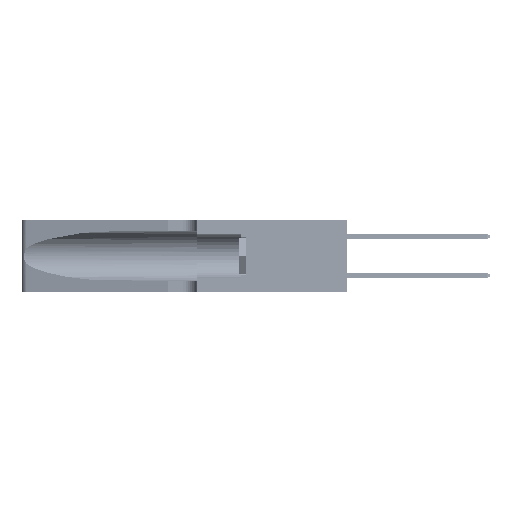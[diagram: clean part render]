
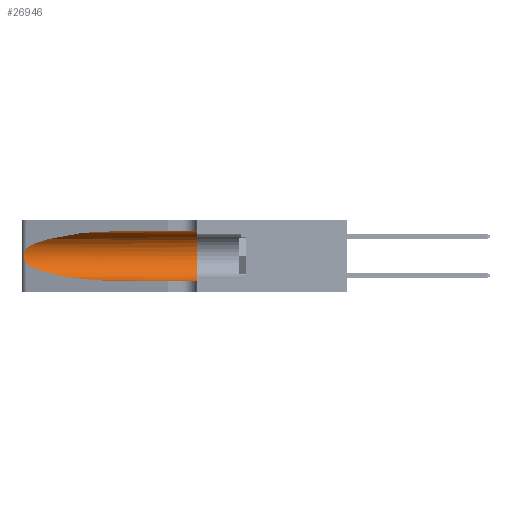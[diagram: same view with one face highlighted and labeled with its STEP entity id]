
A CAD part, left-side view. The second image highlights one B-rep face of the part: STEP entity #26946.
In plain terms, the highlighted cylindrical face has radius 3.308 mm (diameter 6.617 mm), a partial arc.
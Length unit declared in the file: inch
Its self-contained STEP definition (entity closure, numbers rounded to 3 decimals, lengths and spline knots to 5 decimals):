
#239 = VERTEX_POINT ( 'NONE', #35683 ) ;
#592 = CARTESIAN_POINT ( 'NONE',  ( 0.1305, 0.72297, 0.31525 ) ) ;
#1449 = ORIENTED_EDGE ( 'NONE', *, *, #2197, .T. ) ;
#1639 = DIRECTION ( 'NONE',  ( 0., 0., -1. ) ) ;
#1940 = VERTEX_POINT ( 'NONE', #25995 ) ;
#2197 = EDGE_CURVE ( 'NONE', #39018, #12454, #44494, .T. ) ;
#3047 = CARTESIAN_POINT ( 'NONE',  ( 0.25639, 1.23184, 0.21858 ) ) ;
#3977 = CARTESIAN_POINT ( 'NONE',  ( 0.25487, 1.22718, 0.14631 ) ) ;
#7223 = CARTESIAN_POINT ( 'NONE',  ( 0.25854, 1.2359, 0.20912 ) ) ;
#11367 = CARTESIAN_POINT ( 'NONE',  ( 0.26075, 1.23896, 0.19203 ) ) ;
#11879 =( BOUNDED_CURVE ( )  B_SPLINE_CURVE ( 3, ( #39941, #52371, #48402, #23644 ),
 .UNSPECIFIED., .F., .F. ) 
 B_SPLINE_CURVE_WITH_KNOTS ( ( 4, 4 ),
 ( 3.44316, 4.71239 ),
 .UNSPECIFIED. ) 
 CURVE ( )  GEOMETRIC_REPRESENTATION_ITEM ( )  RATIONAL_B_SPLINE_CURVE ( ( 1., 0.87, 0.87, 1. ) ) 
 REPRESENTATION_ITEM ( '' )  );
#12454 = VERTEX_POINT ( 'NONE', #33101 ) ;
#12565 = ORIENTED_EDGE ( 'NONE', *, *, #51630, .F. ) ;
#13204 = AXIS2_PLACEMENT_3D ( 'NONE', #22966, #51884, #27144 ) ;
#14034 = CYLINDRICAL_SURFACE ( 'NONE', #30666, 0.13025 ) ;
#15521 = CARTESIAN_POINT ( 'NONE',  ( 0.26017, 1.23833, 0.17102 ) ) ;
#16497 = CARTESIAN_POINT ( 'NONE',  ( 0.1305, 1.61858, 0.05475 ) ) ;
#18118 = CARTESIAN_POINT ( 'NONE',  ( 0.1305, 1.61858, 0.185 ) ) ;
#19456 = CARTESIAN_POINT ( 'NONE',  ( 0.1305, 0.72297, 0.31525 ) ) ;
#19464 = CARTESIAN_POINT ( 'NONE',  ( 0.25555, 1.22994, 0.2215 ) ) ;
#19646 = CARTESIAN_POINT ( 'NONE',  ( 0.25789, 1.23486, 0.15765 ) ) ;
#19848 = DIRECTION ( 'NONE',  ( 0., -1., 0. ) ) ;
#21571 = ORIENTED_EDGE ( 'NONE', *, *, #47830, .F. ) ;
#22966 = CARTESIAN_POINT ( 'NONE',  ( 0.1305, 0.35, 0.185 ) ) ;
#23084 = B_SPLINE_CURVE_WITH_KNOTS ( 'NONE', 3,
 ( #48365, #19464, #3047, #31985, #7223, #36110, #11367, #40264, #15521, #44382, #19646, #48542, #23790, #52678 ),
 .UNSPECIFIED., .F., .F.,
 ( 4, 2, 2, 2, 2, 2, 4 ),
 ( 0., 0.00027, 0.00053, 0.00107, 0.0016, 0.00187, 0.00214 ),
 .UNSPECIFIED. ) ;
#23644 = CARTESIAN_POINT ( 'NONE',  ( 0.1305, 0.72297, 0.05475 ) ) ;
#23790 = CARTESIAN_POINT ( 'NONE',  ( 0.25555, 1.22993, 0.14849 ) ) ;
#25995 = CARTESIAN_POINT ( 'NONE',  ( 0.1305, 0.35, 0.31525 ) ) ;
#26430 = DIRECTION ( 'NONE',  ( 0., -1., 0. ) ) ;
#26946 = ADVANCED_FACE ( 'NONE', ( #37276 ), #14034, .F. ) ;
#27144 = DIRECTION ( 'NONE',  ( 0., 0., 1. ) ) ;
#29186 = EDGE_CURVE ( 'NONE', #12454, #50051, #23084, .T. ) ;
#30012 = VECTOR ( 'NONE', #53472, 39.37008 ) ;
#30666 = AXIS2_PLACEMENT_3D ( 'NONE', #18118, #26430, #1639 ) ;
#31324 = LINE ( 'NONE', #16497, #30012 ) ;
#31796 = CARTESIAN_POINT ( 'NONE',  ( 0.2373, 1.15595, 0.28018 ) ) ;
#31985 = CARTESIAN_POINT ( 'NONE',  ( 0.25787, 1.23484, 0.2124 ) ) ;
#32183 = CARTESIAN_POINT ( 'NONE',  ( 0.1305, 1.61858, 0.31525 ) ) ;
#33101 = CARTESIAN_POINT ( 'NONE',  ( 0.25487, 1.22718, 0.22369 ) ) ;
#33103 = VECTOR ( 'NONE', #19848, 39.37008 ) ;
#33490 = EDGE_LOOP ( 'NONE', ( #1449, #34465, #49319, #40314, #12565, #21571 ) ) ;
#34465 = ORIENTED_EDGE ( 'NONE', *, *, #29186, .T. ) ;
#35683 = CARTESIAN_POINT ( 'NONE',  ( 0.1305, 0.72297, 0.05475 ) ) ;
#36110 = CARTESIAN_POINT ( 'NONE',  ( 0.26018, 1.23835, 0.19895 ) ) ;
#37189 = EDGE_CURVE ( 'NONE', #50051, #239, #11879, .T. ) ;
#37276 = FACE_OUTER_BOUND ( 'NONE', #33490, .T. ) ;
#39018 = VERTEX_POINT ( 'NONE', #592 ) ;
#39941 = CARTESIAN_POINT ( 'NONE',  ( 0.25487, 1.22718, 0.14631 ) ) ;
#40072 = CARTESIAN_POINT ( 'NONE',  ( 0.18966, 0.96281, 0.31525 ) ) ;
#40264 = CARTESIAN_POINT ( 'NONE',  ( 0.26075, 1.23896, 0.178 ) ) ;
#40314 = ORIENTED_EDGE ( 'NONE', *, *, #51920, .T. ) ;
#41977 = CARTESIAN_POINT ( 'NONE',  ( 0.1305, 0.35, 0.05475 ) ) ;
#44021 = LINE ( 'NONE', #32183, #33103 ) ;
#44382 = CARTESIAN_POINT ( 'NONE',  ( 0.25856, 1.23593, 0.16098 ) ) ;
#44494 =( BOUNDED_CURVE ( )  B_SPLINE_CURVE ( 3, ( #19456, #40072, #31796, #48358 ),
 .UNSPECIFIED., .F., .F. ) 
 B_SPLINE_CURVE_WITH_KNOTS ( ( 4, 4 ),
 ( 1.5708, 2.84003 ),
 .UNSPECIFIED. ) 
 CURVE ( )  GEOMETRIC_REPRESENTATION_ITEM ( )  RATIONAL_B_SPLINE_CURVE ( ( 1., 0.87, 0.87, 1. ) ) 
 REPRESENTATION_ITEM ( '' )  );
#46825 = CIRCLE ( 'NONE', #13204, 0.13025 ) ;
#47830 = EDGE_CURVE ( 'NONE', #39018, #1940, #44021, .T. ) ;
#48358 = CARTESIAN_POINT ( 'NONE',  ( 0.25487, 1.22718, 0.22369 ) ) ;
#48365 = CARTESIAN_POINT ( 'NONE',  ( 0.25487, 1.22718, 0.22369 ) ) ;
#48402 = CARTESIAN_POINT ( 'NONE',  ( 0.18966, 0.96281, 0.05475 ) ) ;
#48542 = CARTESIAN_POINT ( 'NONE',  ( 0.25639, 1.23186, 0.15144 ) ) ;
#49319 = ORIENTED_EDGE ( 'NONE', *, *, #37189, .T. ) ;
#50051 = VERTEX_POINT ( 'NONE', #3977 ) ;
#51630 = EDGE_CURVE ( 'NONE', #1940, #53346, #46825, .T. ) ;
#51884 = DIRECTION ( 'NONE',  ( 0., 1., 0. ) ) ;
#51920 = EDGE_CURVE ( 'NONE', #239, #53346, #31324, .T. ) ;
#52371 = CARTESIAN_POINT ( 'NONE',  ( 0.2373, 1.15595, 0.08982 ) ) ;
#52678 = CARTESIAN_POINT ( 'NONE',  ( 0.25487, 1.22718, 0.14631 ) ) ;
#53346 = VERTEX_POINT ( 'NONE', #41977 ) ;
#53472 = DIRECTION ( 'NONE',  ( 0., -1., 0. ) ) ;
